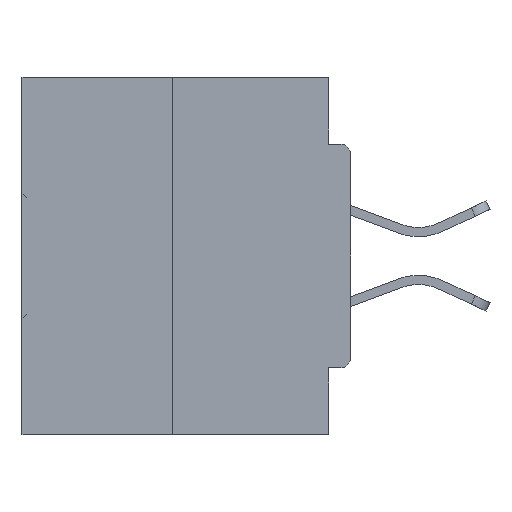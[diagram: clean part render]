
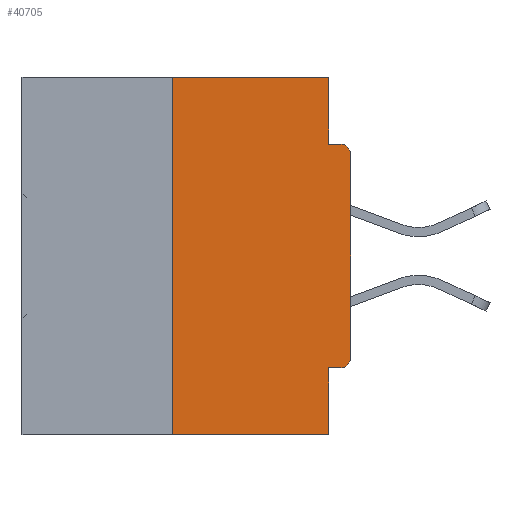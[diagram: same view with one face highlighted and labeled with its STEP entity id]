
A CAD part, left-side view. The second image highlights one B-rep face of the part: STEP entity #40705.
In plain terms, the highlighted planar face has unit normal (-1, 0, 0).
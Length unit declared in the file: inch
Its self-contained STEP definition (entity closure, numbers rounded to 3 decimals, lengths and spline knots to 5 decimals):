
#1038 = CARTESIAN_POINT ( 'NONE',  ( 0., 0., -0.1085 ) ) ;
#1092 = VECTOR ( 'NONE', #2281, 39.37008 ) ;
#2045 = CARTESIAN_POINT ( 'NONE',  ( 0., 0.015, -0.4065 ) ) ;
#2281 = DIRECTION ( 'NONE',  ( 0., 1., 0. ) ) ;
#2830 = AXIS2_PLACEMENT_3D ( 'NONE', #31720, #42303, #32312 ) ;
#3446 = DIRECTION ( 'NONE',  ( 0., 0., 1. ) ) ;
#3476 = CARTESIAN_POINT ( 'NONE',  ( 0., 0.031, -0.5 ) ) ;
#4480 = DIRECTION ( 'NONE',  ( 0., 0., -1. ) ) ;
#5692 = LINE ( 'NONE', #43176, #32876 ) ;
#6529 = LINE ( 'NONE', #30668, #35937 ) ;
#6589 = CARTESIAN_POINT ( 'NONE',  ( 0., 0., 0. ) ) ;
#7681 = EDGE_CURVE ( 'NONE', #39436, #44835, #5692, .T. ) ;
#8006 = ORIENTED_EDGE ( 'NONE', *, *, #31052, .T. ) ;
#8164 = CARTESIAN_POINT ( 'NONE',  ( 0., 0.031, -0.4065 ) ) ;
#8479 = CARTESIAN_POINT ( 'NONE',  ( 0., 0.46, 0. ) ) ;
#8592 = ORIENTED_EDGE ( 'NONE', *, *, #44624, .F. ) ;
#9498 = CIRCLE ( 'NONE', #2830, 0.015 ) ;
#10054 = EDGE_CURVE ( 'NONE', #20507, #44799, #17355, .T. ) ;
#10216 = AXIS2_PLACEMENT_3D ( 'NONE', #29855, #31005, #16553 ) ;
#11882 = DIRECTION ( 'NONE',  ( 0., -1., 0. ) ) ;
#12107 = PLANE ( 'NONE',  #27787 ) ;
#12201 = CARTESIAN_POINT ( 'NONE',  ( 0., 0.031, 0. ) ) ;
#12313 = VECTOR ( 'NONE', #21376, 39.37008 ) ;
#14362 = DIRECTION ( 'NONE',  ( 0., 0., -1. ) ) ;
#14556 = VECTOR ( 'NONE', #14362, 39.37008 ) ;
#14895 = CARTESIAN_POINT ( 'NONE',  ( 0., 0.25, 0. ) ) ;
#15193 = ORIENTED_EDGE ( 'NONE', *, *, #7681, .T. ) ;
#15428 = CARTESIAN_POINT ( 'NONE',  ( 0., 0.031, -0.0935 ) ) ;
#16553 = DIRECTION ( 'NONE',  ( 0., 0., -1. ) ) ;
#17031 = VERTEX_POINT ( 'NONE', #8164 ) ;
#17355 = CIRCLE ( 'NONE', #10216, 0.015 ) ;
#17592 = DIRECTION ( 'NONE',  ( 0., 0., -1. ) ) ;
#18558 = ORIENTED_EDGE ( 'NONE', *, *, #32167, .T. ) ;
#18629 = VERTEX_POINT ( 'NONE', #15428 ) ;
#19505 = ORIENTED_EDGE ( 'NONE', *, *, #10054, .T. ) ;
#20507 = VERTEX_POINT ( 'NONE', #2045 ) ;
#21376 = DIRECTION ( 'NONE',  ( 0., -1., 0. ) ) ;
#21495 = VECTOR ( 'NONE', #17592, 39.37008 ) ;
#22786 = LINE ( 'NONE', #23544, #1092 ) ;
#23254 = VERTEX_POINT ( 'NONE', #1038 ) ;
#23544 = CARTESIAN_POINT ( 'NONE',  ( 0., 0., -0.4065 ) ) ;
#23989 = ORIENTED_EDGE ( 'NONE', *, *, #41422, .F. ) ;
#24471 = CARTESIAN_POINT ( 'NONE',  ( 0., 0.031, -0.5 ) ) ;
#25250 = VECTOR ( 'NONE', #11882, 39.37008 ) ;
#25619 = LINE ( 'NONE', #39077, #12313 ) ;
#25723 = CARTESIAN_POINT ( 'NONE',  ( 0., 0.46, 0. ) ) ;
#26891 = CARTESIAN_POINT ( 'NONE',  ( 0., 0.015, -0.0935 ) ) ;
#27581 = VERTEX_POINT ( 'NONE', #12201 ) ;
#27787 = AXIS2_PLACEMENT_3D ( 'NONE', #25723, #37133, #4480 ) ;
#27909 = EDGE_CURVE ( 'NONE', #39436, #31705, #6529, .T. ) ;
#28303 = EDGE_CURVE ( 'NONE', #17031, #44835, #30964, .T. ) ;
#28677 = DIRECTION ( 'NONE',  ( 0., -1., 0. ) ) ;
#29855 = CARTESIAN_POINT ( 'NONE',  ( 0., 0.015, -0.3915 ) ) ;
#29990 = DIRECTION ( 'NONE',  ( 0., 0., 1. ) ) ;
#30668 = CARTESIAN_POINT ( 'NONE',  ( 0., 0.25, 0. ) ) ;
#30698 = LINE ( 'NONE', #6589, #33432 ) ;
#30785 = ORIENTED_EDGE ( 'NONE', *, *, #30888, .F. ) ;
#30888 = EDGE_CURVE ( 'NONE', #18629, #43466, #25619, .T. ) ;
#30905 = LINE ( 'NONE', #8479, #25250 ) ;
#30964 = LINE ( 'NONE', #3476, #21495 ) ;
#31005 = DIRECTION ( 'NONE',  ( -1., 0., 0. ) ) ;
#31052 = EDGE_CURVE ( 'NONE', #44799, #23254, #30698, .T. ) ;
#31582 = CARTESIAN_POINT ( 'NONE',  ( 0., 0.25, -0.5 ) ) ;
#31705 = VERTEX_POINT ( 'NONE', #14895 ) ;
#31720 = CARTESIAN_POINT ( 'NONE',  ( 0., 0.015, -0.1085 ) ) ;
#32167 = EDGE_CURVE ( 'NONE', #23254, #43466, #9498, .T. ) ;
#32312 = DIRECTION ( 'NONE',  ( 0., 0., -1. ) ) ;
#32876 = VECTOR ( 'NONE', #28677, 39.37008 ) ;
#33098 = ORIENTED_EDGE ( 'NONE', *, *, #42528, .F. ) ;
#33432 = VECTOR ( 'NONE', #3446, 39.37008 ) ;
#33668 = ORIENTED_EDGE ( 'NONE', *, *, #27909, .F. ) ;
#35324 = FACE_OUTER_BOUND ( 'NONE', #42895, .T. ) ;
#35937 = VECTOR ( 'NONE', #29990, 39.37008 ) ;
#37133 = DIRECTION ( 'NONE',  ( 1., 0., 0. ) ) ;
#38363 = CARTESIAN_POINT ( 'NONE',  ( 0., 0., -0.3915 ) ) ;
#39077 = CARTESIAN_POINT ( 'NONE',  ( 0., 0., -0.0935 ) ) ;
#39436 = VERTEX_POINT ( 'NONE', #31582 ) ;
#40705 = ADVANCED_FACE ( 'NONE', ( #35324 ), #12107, .F. ) ;
#41422 = EDGE_CURVE ( 'NONE', #31705, #27581, #30905, .T. ) ;
#42303 = DIRECTION ( 'NONE',  ( -1., 0., 0. ) ) ;
#42356 = ORIENTED_EDGE ( 'NONE', *, *, #28303, .F. ) ;
#42528 = EDGE_CURVE ( 'NONE', #27581, #18629, #42948, .T. ) ;
#42895 = EDGE_LOOP ( 'NONE', ( #23989, #33668, #15193, #42356, #8592, #19505, #8006, #18558, #30785, #33098 ) ) ;
#42948 = LINE ( 'NONE', #43425, #14556 ) ;
#43176 = CARTESIAN_POINT ( 'NONE',  ( 0., 0.46, -0.5 ) ) ;
#43425 = CARTESIAN_POINT ( 'NONE',  ( 0., 0.031, 0. ) ) ;
#43466 = VERTEX_POINT ( 'NONE', #26891 ) ;
#44624 = EDGE_CURVE ( 'NONE', #20507, #17031, #22786, .T. ) ;
#44799 = VERTEX_POINT ( 'NONE', #38363 ) ;
#44835 = VERTEX_POINT ( 'NONE', #24471 ) ;
